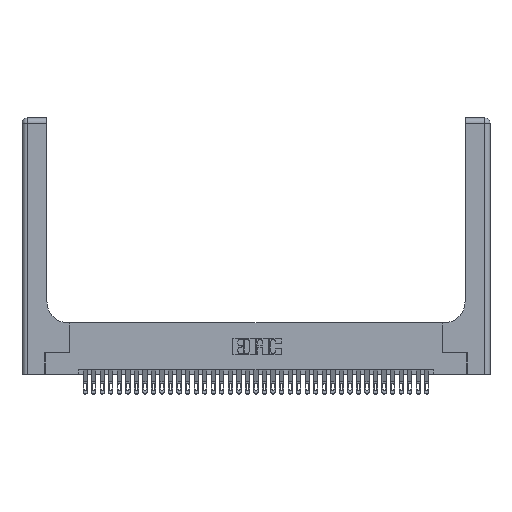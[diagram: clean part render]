
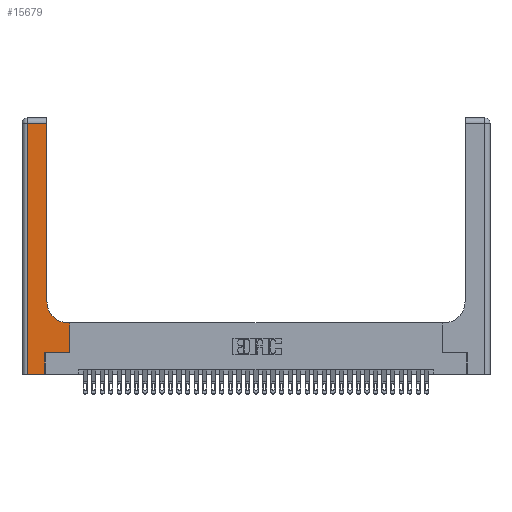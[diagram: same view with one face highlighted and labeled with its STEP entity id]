
A CAD part, top view. The second image highlights one B-rep face of the part: STEP entity #15679.
In plain terms, the highlighted planar face has unit normal (0, 0, 1).
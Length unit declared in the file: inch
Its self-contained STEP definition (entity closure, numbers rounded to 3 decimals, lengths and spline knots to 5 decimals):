
#23 = EDGE_CURVE ( 'NONE', #19446, #15608, #30241, .T. ) ;
#1918 = EDGE_LOOP ( 'NONE', ( #33145, #17813, #29175, #6652, #26516, #34095, #35023, #4857, #24295 ) ) ;
#1922 = DIRECTION ( 'NONE',  ( 0., 0., -1. ) ) ;
#2708 = LINE ( 'NONE', #19096, #17574 ) ;
#2780 = CARTESIAN_POINT ( 'NONE',  ( 0.269, 0., 0.37 ) ) ;
#3518 = VERTEX_POINT ( 'NONE', #16382 ) ;
#3980 = AXIS2_PLACEMENT_3D ( 'NONE', #20797, #29518, #12009 ) ;
#4288 = VECTOR ( 'NONE', #34514, 39.37008 ) ;
#4857 = ORIENTED_EDGE ( 'NONE', *, *, #29434, .T. ) ;
#5159 = CIRCLE ( 'NONE', #14071, 0.25 ) ;
#5459 = CARTESIAN_POINT ( 'NONE',  ( 0.06, 2.94, 0.37 ) ) ;
#6652 = ORIENTED_EDGE ( 'NONE', *, *, #23, .T. ) ;
#6692 = CARTESIAN_POINT ( 'NONE',  ( 0.2915, 2.94, 0.37 ) ) ;
#7024 = CARTESIAN_POINT ( 'NONE',  ( 0.06, 3., 0.37 ) ) ;
#7191 = CARTESIAN_POINT ( 'NONE',  ( 0.5585, 0.25, 0.37 ) ) ;
#8652 = CARTESIAN_POINT ( 'NONE',  ( 0.5585, 0.6, 0.37 ) ) ;
#9024 = PLANE ( 'NONE',  #3980 ) ;
#9655 = LINE ( 'NONE', #27425, #23490 ) ;
#11927 = EDGE_CURVE ( 'NONE', #37811, #19446, #21314, .T. ) ;
#12009 = DIRECTION ( 'NONE',  ( -1., 0., 0. ) ) ;
#12060 = VECTOR ( 'NONE', #35703, 39.37008 ) ;
#12990 = LINE ( 'NONE', #18485, #12060 ) ;
#13008 = DIRECTION ( 'NONE',  ( 0., -1., 0. ) ) ;
#13178 = DIRECTION ( 'NONE',  ( 0., 1., 0. ) ) ;
#13369 = LINE ( 'NONE', #7191, #20305 ) ;
#14071 = AXIS2_PLACEMENT_3D ( 'NONE', #19717, #1922, #22637 ) ;
#15608 = VERTEX_POINT ( 'NONE', #2780 ) ;
#15679 = ADVANCED_FACE ( 'NONE', ( #16540 ), #9024, .F. ) ;
#16382 = CARTESIAN_POINT ( 'NONE',  ( 0.269, 0.25, 0.37 ) ) ;
#16540 = FACE_OUTER_BOUND ( 'NONE', #1918, .T. ) ;
#16804 = VERTEX_POINT ( 'NONE', #24267 ) ;
#17246 = VERTEX_POINT ( 'NONE', #8652 ) ;
#17574 = VECTOR ( 'NONE', #21909, 39.37008 ) ;
#17813 = ORIENTED_EDGE ( 'NONE', *, *, #20301, .T. ) ;
#18100 = CARTESIAN_POINT ( 'NONE',  ( 0.06, 0., 0.37 ) ) ;
#18485 = CARTESIAN_POINT ( 'NONE',  ( 0.269, 0., 0.37 ) ) ;
#19096 = CARTESIAN_POINT ( 'NONE',  ( 0.2915, 0.6, 0.37 ) ) ;
#19364 = CARTESIAN_POINT ( 'NONE',  ( 0.2915, 0.85, 0.37 ) ) ;
#19446 = VERTEX_POINT ( 'NONE', #18100 ) ;
#19717 = CARTESIAN_POINT ( 'NONE',  ( 0.5415, 0.85, 0.37 ) ) ;
#20301 = EDGE_CURVE ( 'NONE', #33712, #37811, #28209, .T. ) ;
#20305 = VECTOR ( 'NONE', #13178, 39.37008 ) ;
#20413 = VECTOR ( 'NONE', #13008, 39.37008 ) ;
#20501 = VECTOR ( 'NONE', #24563, 39.37008 ) ;
#20516 = EDGE_CURVE ( 'NONE', #30032, #25939, #5159, .T. ) ;
#20797 = CARTESIAN_POINT ( 'NONE',  ( 0., 3., 0.37 ) ) ;
#21314 = LINE ( 'NONE', #7024, #20413 ) ;
#21590 = DIRECTION ( 'NONE',  ( 0., 1., 0. ) ) ;
#21632 = CARTESIAN_POINT ( 'NONE',  ( 0., 2.94, 0.37 ) ) ;
#21909 = DIRECTION ( 'NONE',  ( -1., 0., 0. ) ) ;
#22637 = DIRECTION ( 'NONE',  ( 1., 0., 0. ) ) ;
#22796 = CARTESIAN_POINT ( 'NONE',  ( 0.5415, 0.6, 0.37 ) ) ;
#23490 = VECTOR ( 'NONE', #21590, 39.37008 ) ;
#23525 = EDGE_CURVE ( 'NONE', #16804, #17246, #13369, .T. ) ;
#24267 = CARTESIAN_POINT ( 'NONE',  ( 0.5585, 0.25, 0.37 ) ) ;
#24295 = ORIENTED_EDGE ( 'NONE', *, *, #20516, .T. ) ;
#24563 = DIRECTION ( 'NONE',  ( -1., 0., 0. ) ) ;
#25939 = VERTEX_POINT ( 'NONE', #19364 ) ;
#26516 = ORIENTED_EDGE ( 'NONE', *, *, #34214, .T. ) ;
#27425 = CARTESIAN_POINT ( 'NONE',  ( 0.2915, 3., 0.37 ) ) ;
#28209 = LINE ( 'NONE', #21632, #20501 ) ;
#28680 = LINE ( 'NONE', #31685, #4288 ) ;
#29175 = ORIENTED_EDGE ( 'NONE', *, *, #11927, .T. ) ;
#29434 = EDGE_CURVE ( 'NONE', #17246, #30032, #2708, .T. ) ;
#29518 = DIRECTION ( 'NONE',  ( 0., 0., -1. ) ) ;
#30032 = VERTEX_POINT ( 'NONE', #22796 ) ;
#30241 = LINE ( 'NONE', #31469, #37791 ) ;
#31469 = CARTESIAN_POINT ( 'NONE',  ( 0., 0., 0.37 ) ) ;
#31685 = CARTESIAN_POINT ( 'NONE',  ( 0.269, 0.25, 0.37 ) ) ;
#32455 = EDGE_CURVE ( 'NONE', #3518, #16804, #28680, .T. ) ;
#33145 = ORIENTED_EDGE ( 'NONE', *, *, #35416, .T. ) ;
#33712 = VERTEX_POINT ( 'NONE', #6692 ) ;
#34095 = ORIENTED_EDGE ( 'NONE', *, *, #32455, .T. ) ;
#34214 = EDGE_CURVE ( 'NONE', #15608, #3518, #12990, .T. ) ;
#34514 = DIRECTION ( 'NONE',  ( 1., 0., 0. ) ) ;
#35023 = ORIENTED_EDGE ( 'NONE', *, *, #23525, .T. ) ;
#35416 = EDGE_CURVE ( 'NONE', #25939, #33712, #9655, .T. ) ;
#35703 = DIRECTION ( 'NONE',  ( 0., 1., 0. ) ) ;
#37415 = DIRECTION ( 'NONE',  ( 1., 0., 0. ) ) ;
#37791 = VECTOR ( 'NONE', #37415, 39.37008 ) ;
#37811 = VERTEX_POINT ( 'NONE', #5459 ) ;
